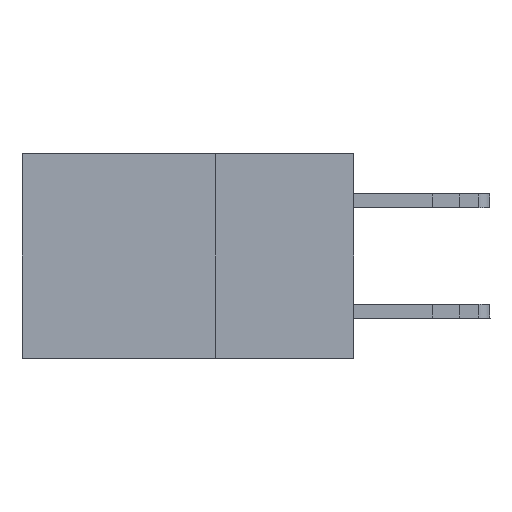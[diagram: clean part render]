
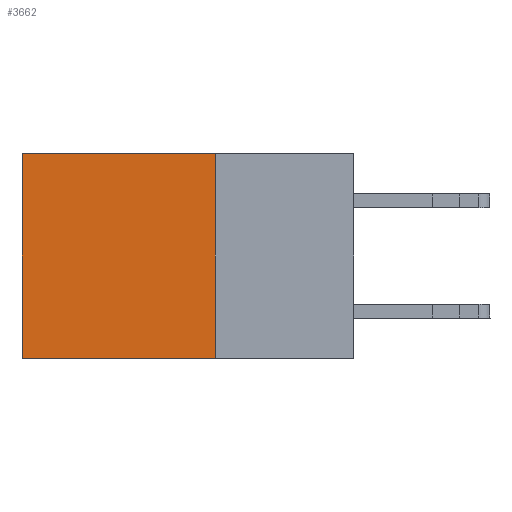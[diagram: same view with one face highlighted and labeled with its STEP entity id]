
A CAD part, left-side view. The second image highlights one B-rep face of the part: STEP entity #3662.
In plain terms, the highlighted planar face has unit normal (-1, 0, 0).
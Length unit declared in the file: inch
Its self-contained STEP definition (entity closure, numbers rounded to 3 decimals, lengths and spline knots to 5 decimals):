
#291 = ORIENTED_EDGE ( 'NONE', *, *, #9293, .T. ) ;
#748 = VERTEX_POINT ( 'NONE', #18437 ) ;
#1067 = CARTESIAN_POINT ( 'NONE',  ( 0.2875, 0.6, -0.37 ) ) ;
#3187 = VECTOR ( 'NONE', #13363, 39.37008 ) ;
#3662 = ADVANCED_FACE ( 'NONE', ( #17134 ), #14693, .F. ) ;
#4840 = ORIENTED_EDGE ( 'NONE', *, *, #8902, .F. ) ;
#5650 = DIRECTION ( 'NONE',  ( 1., 0., 0. ) ) ;
#5802 = CARTESIAN_POINT ( 'NONE',  ( 0.2875, 0.6, 0. ) ) ;
#6566 = VERTEX_POINT ( 'NONE', #28174 ) ;
#6797 = VECTOR ( 'NONE', #27125, 39.37008 ) ;
#7084 = VERTEX_POINT ( 'NONE', #1067 ) ;
#8734 = VECTOR ( 'NONE', #17394, 39.37008 ) ;
#8902 = EDGE_CURVE ( 'NONE', #23084, #7084, #22914, .T. ) ;
#9293 = EDGE_CURVE ( 'NONE', #6566, #7084, #27375, .T. ) ;
#12717 = CARTESIAN_POINT ( 'NONE',  ( 0.2875, 0.25, 0. ) ) ;
#12823 = DIRECTION ( 'NONE',  ( 0., 0., -1. ) ) ;
#13363 = DIRECTION ( 'NONE',  ( 0., 1., 0. ) ) ;
#14693 = PLANE ( 'NONE',  #19356 ) ;
#15124 = CARTESIAN_POINT ( 'NONE',  ( 0.2875, 0.25, -0.37 ) ) ;
#16524 = VECTOR ( 'NONE', #27280, 39.37008 ) ;
#17134 = FACE_OUTER_BOUND ( 'NONE', #21863, .T. ) ;
#17208 = ORIENTED_EDGE ( 'NONE', *, *, #29747, .F. ) ;
#17394 = DIRECTION ( 'NONE',  ( 0., 1., 0. ) ) ;
#18317 = EDGE_CURVE ( 'NONE', #748, #6566, #25535, .T. ) ;
#18437 = CARTESIAN_POINT ( 'NONE',  ( 0.2875, 0.25, 0. ) ) ;
#18728 = ORIENTED_EDGE ( 'NONE', *, *, #18317, .T. ) ;
#19356 = AXIS2_PLACEMENT_3D ( 'NONE', #12717, #5650, #12823 ) ;
#19846 = LINE ( 'NONE', #22233, #6797 ) ;
#21863 = EDGE_LOOP ( 'NONE', ( #291, #4840, #17208, #18728 ) ) ;
#22233 = CARTESIAN_POINT ( 'NONE',  ( 0.2875, 0.25, 0. ) ) ;
#22914 = LINE ( 'NONE', #15124, #8734 ) ;
#23084 = VERTEX_POINT ( 'NONE', #27156 ) ;
#25535 = LINE ( 'NONE', #29657, #3187 ) ;
#27125 = DIRECTION ( 'NONE',  ( 0., 0., -1. ) ) ;
#27156 = CARTESIAN_POINT ( 'NONE',  ( 0.2875, 0.25, -0.37 ) ) ;
#27280 = DIRECTION ( 'NONE',  ( 0., 0., -1. ) ) ;
#27375 = LINE ( 'NONE', #5802, #16524 ) ;
#28174 = CARTESIAN_POINT ( 'NONE',  ( 0.2875, 0.6, 0. ) ) ;
#29657 = CARTESIAN_POINT ( 'NONE',  ( 0.2875, 0.25, 0. ) ) ;
#29747 = EDGE_CURVE ( 'NONE', #748, #23084, #19846, .T. ) ;
